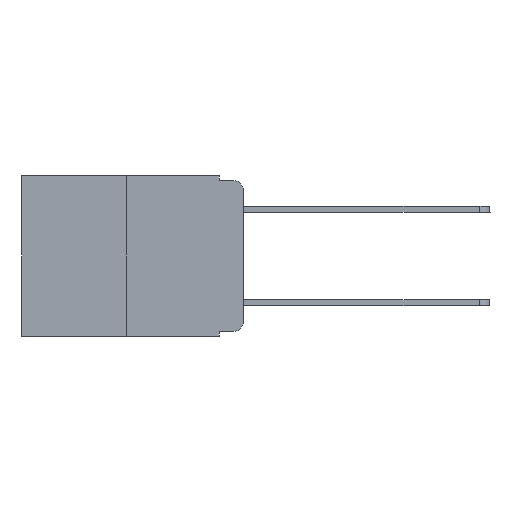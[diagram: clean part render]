
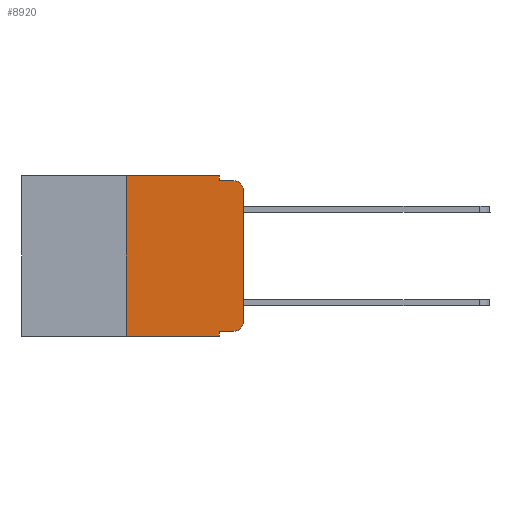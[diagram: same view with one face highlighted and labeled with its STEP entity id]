
A CAD part, left-side view. The second image highlights one B-rep face of the part: STEP entity #8920.
In plain terms, the highlighted planar face has unit normal (-1, 0, 0).
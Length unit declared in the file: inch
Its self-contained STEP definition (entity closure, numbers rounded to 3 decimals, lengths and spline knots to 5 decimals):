
#73 = EDGE_CURVE ( 'NONE', #13860, #7963, #3305, .T. ) ;
#445 = VERTEX_POINT ( 'NONE', #16627 ) ;
#1172 = VECTOR ( 'NONE', #14501, 39.37008 ) ;
#1260 = DIRECTION ( 'NONE',  ( 0., 0., 1. ) ) ;
#1261 = VERTEX_POINT ( 'NONE', #4310 ) ;
#1553 = CARTESIAN_POINT ( 'NONE',  ( 0., 0.02, -0.03 ) ) ;
#1665 = LINE ( 'NONE', #1853, #3904 ) ;
#1691 = VECTOR ( 'NONE', #15651, 39.37008 ) ;
#1694 = CARTESIAN_POINT ( 'NONE',  ( 0., 0.02, -0.313 ) ) ;
#1743 = VERTEX_POINT ( 'NONE', #7215 ) ;
#1815 = ORIENTED_EDGE ( 'NONE', *, *, #14641, .T. ) ;
#1853 = CARTESIAN_POINT ( 'NONE',  ( 0., 0.051, -0.01 ) ) ;
#1924 = DIRECTION ( 'NONE',  ( 0., 0., 1. ) ) ;
#1954 = AXIS2_PLACEMENT_3D ( 'NONE', #1694, #6014, #13171 ) ;
#2259 = DIRECTION ( 'NONE',  ( 0., 0., -1. ) ) ;
#2347 = CARTESIAN_POINT ( 'NONE',  ( 0., 0.25, -0.343 ) ) ;
#2372 = LINE ( 'NONE', #16241, #17883 ) ;
#2651 = ORIENTED_EDGE ( 'NONE', *, *, #4269, .F. ) ;
#2884 = AXIS2_PLACEMENT_3D ( 'NONE', #6942, #5438, #18404 ) ;
#3052 = VECTOR ( 'NONE', #12260, 39.37008 ) ;
#3220 = VECTOR ( 'NONE', #2259, 39.37008 ) ;
#3305 = LINE ( 'NONE', #5388, #12464 ) ;
#3315 = DIRECTION ( 'NONE',  ( 0., -1., 0. ) ) ;
#3589 = CARTESIAN_POINT ( 'NONE',  ( 0., 0.051, 0. ) ) ;
#3749 = CARTESIAN_POINT ( 'NONE',  ( 0., 0., -0.03 ) ) ;
#3869 = LINE ( 'NONE', #14617, #1172 ) ;
#3904 = VECTOR ( 'NONE', #3315, 39.37008 ) ;
#4003 = EDGE_LOOP ( 'NONE', ( #6258, #7113, #2651, #16585, #18409, #7455, #8842, #4650, #1815, #7683 ) ) ;
#4162 = CARTESIAN_POINT ( 'NONE',  ( 0., 0.02, -0.333 ) ) ;
#4199 = DIRECTION ( 'NONE',  ( 0., 0., -1. ) ) ;
#4269 = EDGE_CURVE ( 'NONE', #8802, #10254, #1665, .T. ) ;
#4280 = CARTESIAN_POINT ( 'NONE',  ( 0., 0.051, -0.01 ) ) ;
#4310 = CARTESIAN_POINT ( 'NONE',  ( 0., 0.051, 0. ) ) ;
#4650 = ORIENTED_EDGE ( 'NONE', *, *, #18192, .F. ) ;
#4878 = DIRECTION ( 'NONE',  ( 0., 0., -1. ) ) ;
#5388 = CARTESIAN_POINT ( 'NONE',  ( 0., 0., 0. ) ) ;
#5438 = DIRECTION ( 'NONE',  ( 1., 0., 0. ) ) ;
#5720 = CIRCLE ( 'NONE', #1954, 0.02 ) ;
#6014 = DIRECTION ( 'NONE',  ( -1., 0., 0. ) ) ;
#6258 = ORIENTED_EDGE ( 'NONE', *, *, #73, .T. ) ;
#6273 = EDGE_CURVE ( 'NONE', #15407, #445, #15965, .T. ) ;
#6278 = VECTOR ( 'NONE', #1924, 39.37008 ) ;
#6919 = VERTEX_POINT ( 'NONE', #11610 ) ;
#6942 = CARTESIAN_POINT ( 'NONE',  ( 0., 0.473, 0. ) ) ;
#7113 = ORIENTED_EDGE ( 'NONE', *, *, #16752, .T. ) ;
#7215 = CARTESIAN_POINT ( 'NONE',  ( 0., 0.051, -0.333 ) ) ;
#7383 = AXIS2_PLACEMENT_3D ( 'NONE', #1553, #11560, #4199 ) ;
#7455 = ORIENTED_EDGE ( 'NONE', *, *, #6273, .F. ) ;
#7552 = CARTESIAN_POINT ( 'NONE',  ( 0., 0.25, 0. ) ) ;
#7577 = CARTESIAN_POINT ( 'NONE',  ( 0., 0.02, -0.01 ) ) ;
#7683 = ORIENTED_EDGE ( 'NONE', *, *, #13795, .T. ) ;
#7963 = VERTEX_POINT ( 'NONE', #3749 ) ;
#8153 = CIRCLE ( 'NONE', #7383, 0.02 ) ;
#8802 = VERTEX_POINT ( 'NONE', #4280 ) ;
#8836 = VERTEX_POINT ( 'NONE', #4162 ) ;
#8842 = ORIENTED_EDGE ( 'NONE', *, *, #16345, .T. ) ;
#8920 = ADVANCED_FACE ( 'NONE', ( #11464 ), #10083, .F. ) ;
#10083 = PLANE ( 'NONE',  #2884 ) ;
#10209 = LINE ( 'NONE', #14262, #1691 ) ;
#10254 = VERTEX_POINT ( 'NONE', #7577 ) ;
#11464 = FACE_OUTER_BOUND ( 'NONE', #4003, .T. ) ;
#11560 = DIRECTION ( 'NONE',  ( -1., 0., 0. ) ) ;
#11610 = CARTESIAN_POINT ( 'NONE',  ( 0., 0.051, -0.343 ) ) ;
#12260 = DIRECTION ( 'NONE',  ( 0., -1., 0. ) ) ;
#12464 = VECTOR ( 'NONE', #1260, 39.37008 ) ;
#13171 = DIRECTION ( 'NONE',  ( 0., 0., -1. ) ) ;
#13607 = EDGE_CURVE ( 'NONE', #445, #1261, #10209, .T. ) ;
#13795 = EDGE_CURVE ( 'NONE', #8836, #13860, #5720, .T. ) ;
#13851 = CARTESIAN_POINT ( 'NONE',  ( 0., 0.051, -0.333 ) ) ;
#13860 = VERTEX_POINT ( 'NONE', #17545 ) ;
#14262 = CARTESIAN_POINT ( 'NONE',  ( 0., 0.473, 0. ) ) ;
#14501 = DIRECTION ( 'NONE',  ( 0., -1., 0. ) ) ;
#14617 = CARTESIAN_POINT ( 'NONE',  ( 0., 0.473, -0.343 ) ) ;
#14641 = EDGE_CURVE ( 'NONE', #1743, #8836, #18319, .T. ) ;
#15407 = VERTEX_POINT ( 'NONE', #2347 ) ;
#15651 = DIRECTION ( 'NONE',  ( 0., -1., 0. ) ) ;
#15965 = LINE ( 'NONE', #7552, #6278 ) ;
#16221 = LINE ( 'NONE', #3589, #3220 ) ;
#16241 = CARTESIAN_POINT ( 'NONE',  ( 0., 0.051, 0. ) ) ;
#16345 = EDGE_CURVE ( 'NONE', #15407, #6919, #3869, .T. ) ;
#16500 = EDGE_CURVE ( 'NONE', #1261, #8802, #2372, .T. ) ;
#16585 = ORIENTED_EDGE ( 'NONE', *, *, #16500, .F. ) ;
#16627 = CARTESIAN_POINT ( 'NONE',  ( 0., 0.25, 0. ) ) ;
#16752 = EDGE_CURVE ( 'NONE', #7963, #10254, #8153, .T. ) ;
#17545 = CARTESIAN_POINT ( 'NONE',  ( 0., 0., -0.313 ) ) ;
#17883 = VECTOR ( 'NONE', #4878, 39.37008 ) ;
#18192 = EDGE_CURVE ( 'NONE', #1743, #6919, #16221, .T. ) ;
#18319 = LINE ( 'NONE', #13851, #3052 ) ;
#18404 = DIRECTION ( 'NONE',  ( 0., 0., -1. ) ) ;
#18409 = ORIENTED_EDGE ( 'NONE', *, *, #13607, .F. ) ;
